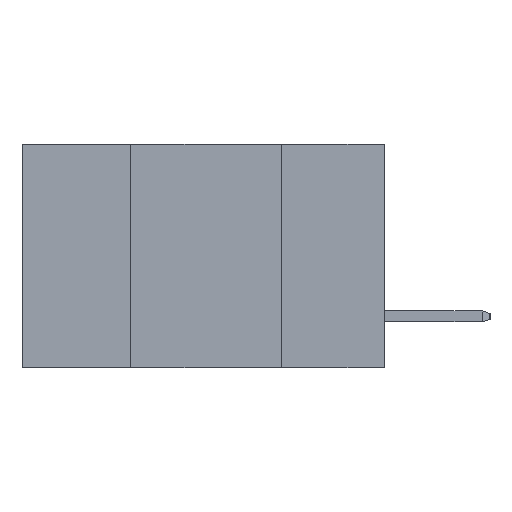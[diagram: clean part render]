
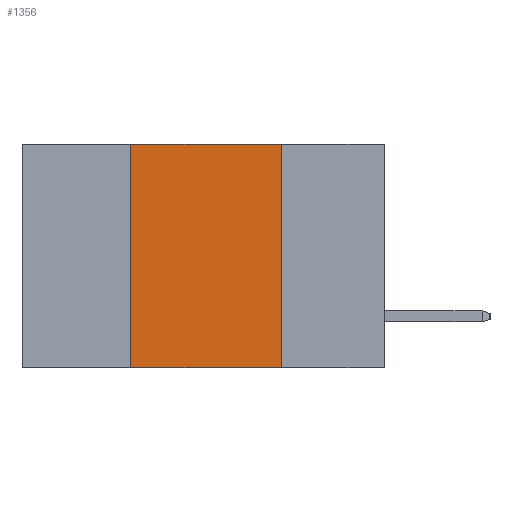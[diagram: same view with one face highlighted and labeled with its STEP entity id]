
A CAD part, left-side view. The second image highlights one B-rep face of the part: STEP entity #1356.
In plain terms, the highlighted planar face has unit normal (-1, 0, 0).
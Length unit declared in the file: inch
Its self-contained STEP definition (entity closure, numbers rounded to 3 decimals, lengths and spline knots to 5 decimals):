
#297 = CARTESIAN_POINT ( 'NONE',  ( 0., 0.42, 0. ) ) ;
#370 = DIRECTION ( 'NONE',  ( 0., -1., 0. ) ) ;
#764 = VERTEX_POINT ( 'NONE', #7971 ) ;
#819 = EDGE_LOOP ( 'NONE', ( #1640, #4736, #2091, #8826 ) ) ;
#1238 = AXIS2_PLACEMENT_3D ( 'NONE', #4018, #2996, #2617 ) ;
#1356 = ADVANCED_FACE ( 'NONE', ( #5436 ), #4670, .F. ) ;
#1640 = ORIENTED_EDGE ( 'NONE', *, *, #6604, .F. ) ;
#1857 = EDGE_CURVE ( 'NONE', #6137, #8965, #4447, .T. ) ;
#2091 = ORIENTED_EDGE ( 'NONE', *, *, #5286, .F. ) ;
#2346 = CARTESIAN_POINT ( 'NONE',  ( 0., 0.17, 0. ) ) ;
#2617 = DIRECTION ( 'NONE',  ( 0., 0., -1. ) ) ;
#2765 = LINE ( 'NONE', #8117, #8205 ) ;
#2996 = DIRECTION ( 'NONE',  ( 1., 0., 0. ) ) ;
#3947 = DIRECTION ( 'NONE',  ( 0., 0., -1. ) ) ;
#4018 = CARTESIAN_POINT ( 'NONE',  ( 0., 0.6, 0. ) ) ;
#4144 = DIRECTION ( 'NONE',  ( 0., -1., 0. ) ) ;
#4447 = LINE ( 'NONE', #4641, #5441 ) ;
#4641 = CARTESIAN_POINT ( 'NONE',  ( 0., 0.6, 0. ) ) ;
#4670 = PLANE ( 'NONE',  #1238 ) ;
#4736 = ORIENTED_EDGE ( 'NONE', *, *, #1857, .F. ) ;
#5078 = LINE ( 'NONE', #8923, #8527 ) ;
#5286 = EDGE_CURVE ( 'NONE', #8113, #6137, #5078, .T. ) ;
#5436 = FACE_OUTER_BOUND ( 'NONE', #819, .T. ) ;
#5441 = VECTOR ( 'NONE', #4144, 39.37008 ) ;
#5909 = LINE ( 'NONE', #6395, #9140 ) ;
#5926 = CARTESIAN_POINT ( 'NONE',  ( 0., 0.42, -0.37 ) ) ;
#6137 = VERTEX_POINT ( 'NONE', #297 ) ;
#6395 = CARTESIAN_POINT ( 'NONE',  ( 0., 0.6, -0.37 ) ) ;
#6604 = EDGE_CURVE ( 'NONE', #8965, #764, #2765, .T. ) ;
#7971 = CARTESIAN_POINT ( 'NONE',  ( 0., 0.17, -0.37 ) ) ;
#8113 = VERTEX_POINT ( 'NONE', #5926 ) ;
#8117 = CARTESIAN_POINT ( 'NONE',  ( 0., 0.17, -0.37 ) ) ;
#8205 = VECTOR ( 'NONE', #3947, 39.37008 ) ;
#8527 = VECTOR ( 'NONE', #8956, 39.37008 ) ;
#8826 = ORIENTED_EDGE ( 'NONE', *, *, #9505, .T. ) ;
#8923 = CARTESIAN_POINT ( 'NONE',  ( 0., 0.42, -0.37 ) ) ;
#8956 = DIRECTION ( 'NONE',  ( 0., 0., 1. ) ) ;
#8965 = VERTEX_POINT ( 'NONE', #2346 ) ;
#9140 = VECTOR ( 'NONE', #370, 39.37008 ) ;
#9505 = EDGE_CURVE ( 'NONE', #8113, #764, #5909, .T. ) ;
